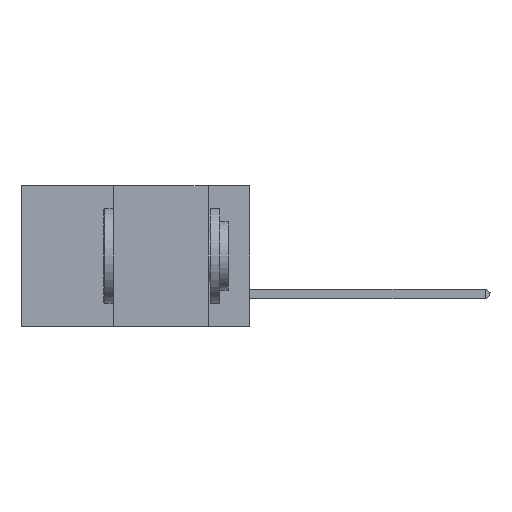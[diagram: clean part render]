
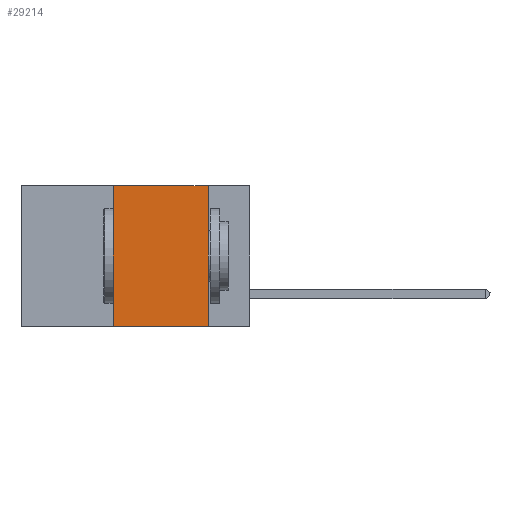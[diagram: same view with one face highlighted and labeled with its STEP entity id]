
A CAD part, left-side view. The second image highlights one B-rep face of the part: STEP entity #29214.
In plain terms, the highlighted planar face has unit normal (-1, 0, 0).
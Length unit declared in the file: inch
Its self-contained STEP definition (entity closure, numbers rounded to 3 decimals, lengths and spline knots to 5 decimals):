
#1250 = VECTOR ( 'NONE', #14229, 39.37008 ) ;
#1484 = EDGE_CURVE ( 'NONE', #31092, #21369, #13559, .T. ) ;
#2213 = CARTESIAN_POINT ( 'NONE',  ( 0., 0.6, 0. ) ) ;
#2442 = EDGE_CURVE ( 'NONE', #6138, #21369, #11645, .T. ) ;
#4795 = VERTEX_POINT ( 'NONE', #15760 ) ;
#4971 = ORIENTED_EDGE ( 'NONE', *, *, #8483, .F. ) ;
#5209 = DIRECTION ( 'NONE',  ( 0., 0., -1. ) ) ;
#6138 = VERTEX_POINT ( 'NONE', #27338 ) ;
#8483 = EDGE_CURVE ( 'NONE', #4795, #6138, #11278, .T. ) ;
#11278 = LINE ( 'NONE', #17426, #27094 ) ;
#11645 = LINE ( 'NONE', #25105, #16301 ) ;
#11802 = ORIENTED_EDGE ( 'NONE', *, *, #2442, .F. ) ;
#11866 = EDGE_CURVE ( 'NONE', #31092, #4795, #32940, .T. ) ;
#12959 = CARTESIAN_POINT ( 'NONE',  ( 0., 0.36, -0.37 ) ) ;
#13559 = LINE ( 'NONE', #35816, #29891 ) ;
#14229 = DIRECTION ( 'NONE',  ( 0., 0., 1. ) ) ;
#15760 = CARTESIAN_POINT ( 'NONE',  ( 0., 0.36, 0. ) ) ;
#16301 = VECTOR ( 'NONE', #22371, 39.37008 ) ;
#16379 = FACE_OUTER_BOUND ( 'NONE', #31079, .T. ) ;
#17426 = CARTESIAN_POINT ( 'NONE',  ( 0., 0.6, 0. ) ) ;
#17854 = DIRECTION ( 'NONE',  ( 0., -1., 0. ) ) ;
#20196 = PLANE ( 'NONE',  #34513 ) ;
#21369 = VERTEX_POINT ( 'NONE', #38437 ) ;
#22371 = DIRECTION ( 'NONE',  ( 0., 0., -1. ) ) ;
#23057 = DIRECTION ( 'NONE',  ( 1., 0., 0. ) ) ;
#25105 = CARTESIAN_POINT ( 'NONE',  ( 0., 0.11, 0. ) ) ;
#27094 = VECTOR ( 'NONE', #34872, 39.37008 ) ;
#27338 = CARTESIAN_POINT ( 'NONE',  ( 0., 0.11, 0. ) ) ;
#27842 = ORIENTED_EDGE ( 'NONE', *, *, #1484, .T. ) ;
#29069 = CARTESIAN_POINT ( 'NONE',  ( 0., 0.36, 0. ) ) ;
#29214 = ADVANCED_FACE ( 'NONE', ( #16379 ), #20196, .F. ) ;
#29891 = VECTOR ( 'NONE', #17854, 39.37008 ) ;
#31079 = EDGE_LOOP ( 'NONE', ( #11802, #4971, #34884, #27842 ) ) ;
#31092 = VERTEX_POINT ( 'NONE', #12959 ) ;
#32940 = LINE ( 'NONE', #29069, #1250 ) ;
#34513 = AXIS2_PLACEMENT_3D ( 'NONE', #2213, #23057, #5209 ) ;
#34872 = DIRECTION ( 'NONE',  ( 0., -1., 0. ) ) ;
#34884 = ORIENTED_EDGE ( 'NONE', *, *, #11866, .F. ) ;
#35816 = CARTESIAN_POINT ( 'NONE',  ( 0., 0.6, -0.37 ) ) ;
#38437 = CARTESIAN_POINT ( 'NONE',  ( 0., 0.11, -0.37 ) ) ;
